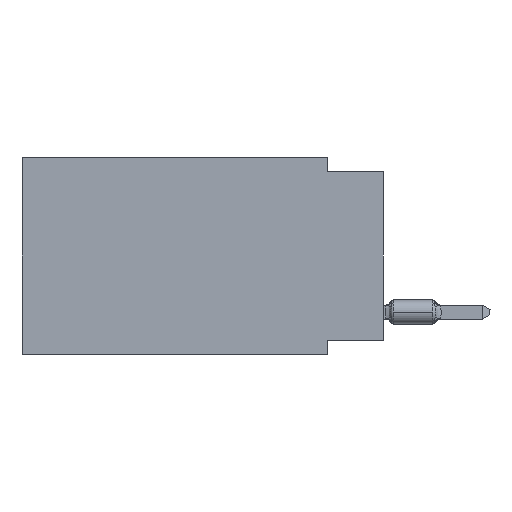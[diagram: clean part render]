
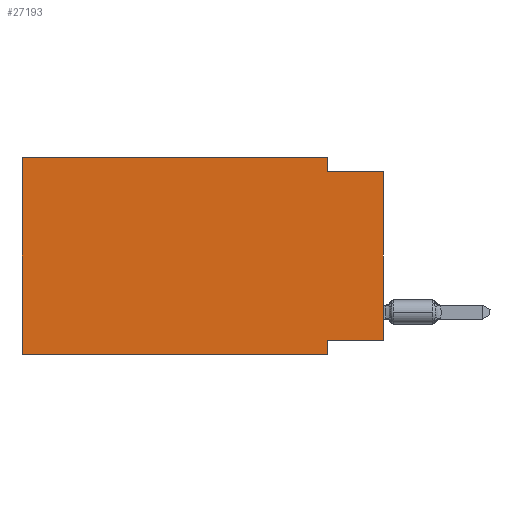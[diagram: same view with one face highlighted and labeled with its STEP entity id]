
A CAD part, left-side view. The second image highlights one B-rep face of the part: STEP entity #27193.
In plain terms, the highlighted planar face has unit normal (-1, 0, 0).
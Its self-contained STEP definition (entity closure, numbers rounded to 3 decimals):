
#424 = VERTEX_POINT ( 'NONE', #24898 ) ;
#1984 = CARTESIAN_POINT ( 'NONE',  ( 0., 2.54, 0. ) ) ;
#2366 = VERTEX_POINT ( 'NONE', #22143 ) ;
#3558 = DIRECTION ( 'NONE',  ( 0., -1., 0. ) ) ;
#3873 = DIRECTION ( 'NONE',  ( 0., -1., 0. ) ) ;
#3944 = CARTESIAN_POINT ( 'NONE',  ( 0., 16.383, 0. ) ) ;
#4269 = DIRECTION ( 'NONE',  ( 0., 1., 0. ) ) ;
#4418 = CARTESIAN_POINT ( 'NONE',  ( 0., 16.383, 0. ) ) ;
#4459 = CARTESIAN_POINT ( 'NONE',  ( 0., 16.383, -8.89 ) ) ;
#5320 = DIRECTION ( 'NONE',  ( 0., 0., -1. ) ) ;
#5373 = LINE ( 'NONE', #23203, #27615 ) ;
#6680 = ORIENTED_EDGE ( 'NONE', *, *, #30497, .F. ) ;
#6706 = VERTEX_POINT ( 'NONE', #17948 ) ;
#7141 = LINE ( 'NONE', #9264, #12340 ) ;
#7264 = VERTEX_POINT ( 'NONE', #4418 ) ;
#7755 = PLANE ( 'NONE',  #25354 ) ;
#8052 = EDGE_CURVE ( 'NONE', #424, #2366, #16942, .T. ) ;
#8460 = CARTESIAN_POINT ( 'NONE',  ( 0., 0., -8.255 ) ) ;
#9264 = CARTESIAN_POINT ( 'NONE',  ( 0., 0., -0.635 ) ) ;
#11643 = LINE ( 'NONE', #31416, #29214 ) ;
#12340 = VECTOR ( 'NONE', #24163, 1000. ) ;
#12755 = ORIENTED_EDGE ( 'NONE', *, *, #17648, .F. ) ;
#13141 = DIRECTION ( 'NONE',  ( 0., 0., -1. ) ) ;
#15255 = DIRECTION ( 'NONE',  ( 0., 0., 1. ) ) ;
#15936 = CARTESIAN_POINT ( 'NONE',  ( 0., 0., -8.255 ) ) ;
#16427 = ORIENTED_EDGE ( 'NONE', *, *, #8052, .T. ) ;
#16590 = DIRECTION ( 'NONE',  ( 0., 0., 1. ) ) ;
#16942 = LINE ( 'NONE', #4459, #17537 ) ;
#17002 = VECTOR ( 'NONE', #13141, 1000. ) ;
#17044 = DIRECTION ( 'NONE',  ( 0., 0., -1. ) ) ;
#17537 = VECTOR ( 'NONE', #3558, 1000. ) ;
#17565 = VERTEX_POINT ( 'NONE', #8460 ) ;
#17640 = CARTESIAN_POINT ( 'NONE',  ( 0., 16.383, 0. ) ) ;
#17648 = EDGE_CURVE ( 'NONE', #6706, #29547, #7141, .T. ) ;
#17931 = CARTESIAN_POINT ( 'NONE',  ( 0., 2.54, -8.255 ) ) ;
#17948 = CARTESIAN_POINT ( 'NONE',  ( 0., 2.54, -0.635 ) ) ;
#18038 = CARTESIAN_POINT ( 'NONE',  ( 0., 2.54, 0. ) ) ;
#19312 = EDGE_CURVE ( 'NONE', #424, #7264, #21115, .T. ) ;
#20073 = VECTOR ( 'NONE', #17044, 1000. ) ;
#20794 = EDGE_CURVE ( 'NONE', #17565, #29547, #5373, .T. ) ;
#21115 = LINE ( 'NONE', #3944, #27178 ) ;
#21145 = ORIENTED_EDGE ( 'NONE', *, *, #31912, .F. ) ;
#21208 = VECTOR ( 'NONE', #4269, 1000. ) ;
#21440 = EDGE_CURVE ( 'NONE', #7264, #28023, #11643, .T. ) ;
#21695 = VERTEX_POINT ( 'NONE', #17931 ) ;
#22143 = CARTESIAN_POINT ( 'NONE',  ( 0., 2.54, -8.89 ) ) ;
#22445 = ORIENTED_EDGE ( 'NONE', *, *, #21440, .F. ) ;
#22818 = EDGE_CURVE ( 'NONE', #28023, #6706, #24173, .T. ) ;
#23203 = CARTESIAN_POINT ( 'NONE',  ( 0., 0., 0. ) ) ;
#24163 = DIRECTION ( 'NONE',  ( 0., -1., 0. ) ) ;
#24173 = LINE ( 'NONE', #1984, #20073 ) ;
#24898 = CARTESIAN_POINT ( 'NONE',  ( 0., 16.383, -8.89 ) ) ;
#25354 = AXIS2_PLACEMENT_3D ( 'NONE', #17640, #27520, #5320 ) ;
#25936 = EDGE_LOOP ( 'NONE', ( #31713, #12755, #31734, #22445, #28939, #16427, #6680, #21145 ) ) ;
#25979 = LINE ( 'NONE', #15936, #21208 ) ;
#27178 = VECTOR ( 'NONE', #16590, 1000. ) ;
#27193 = ADVANCED_FACE ( 'NONE', ( #29966 ), #7755, .F. ) ;
#27520 = DIRECTION ( 'NONE',  ( 1., 0., 0. ) ) ;
#27615 = VECTOR ( 'NONE', #15255, 1000. ) ;
#27886 = CARTESIAN_POINT ( 'NONE',  ( 0., 2.54, -8.89 ) ) ;
#28023 = VERTEX_POINT ( 'NONE', #18038 ) ;
#28939 = ORIENTED_EDGE ( 'NONE', *, *, #19312, .F. ) ;
#29214 = VECTOR ( 'NONE', #3873, 1000. ) ;
#29547 = VERTEX_POINT ( 'NONE', #30797 ) ;
#29966 = FACE_OUTER_BOUND ( 'NONE', #25936, .T. ) ;
#30497 = EDGE_CURVE ( 'NONE', #21695, #2366, #30648, .T. ) ;
#30648 = LINE ( 'NONE', #27886, #17002 ) ;
#30797 = CARTESIAN_POINT ( 'NONE',  ( 0., 0., -0.635 ) ) ;
#31416 = CARTESIAN_POINT ( 'NONE',  ( 0., 16.383, 0. ) ) ;
#31713 = ORIENTED_EDGE ( 'NONE', *, *, #20794, .T. ) ;
#31734 = ORIENTED_EDGE ( 'NONE', *, *, #22818, .F. ) ;
#31912 = EDGE_CURVE ( 'NONE', #17565, #21695, #25979, .T. ) ;
